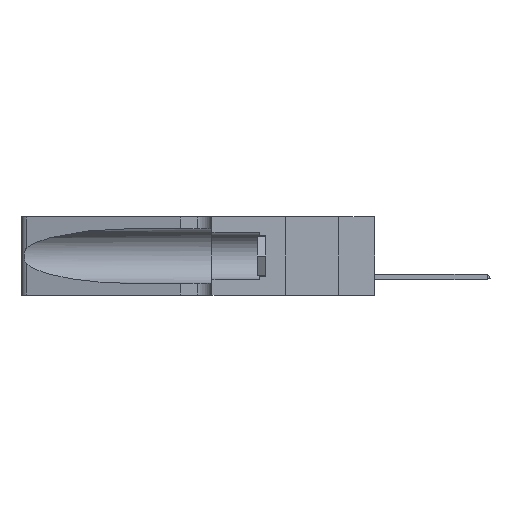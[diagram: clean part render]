
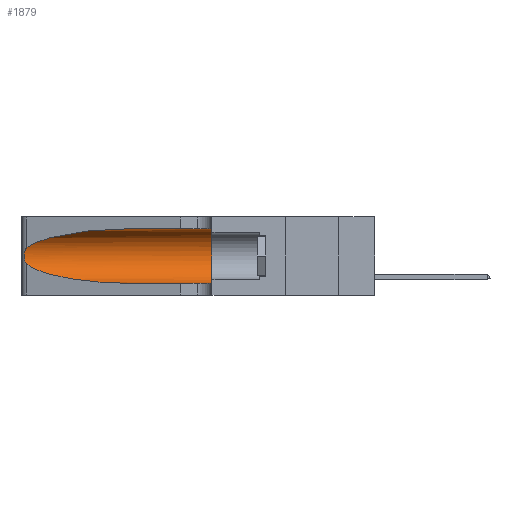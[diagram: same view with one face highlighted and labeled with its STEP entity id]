
A CAD part, left-side view. The second image highlights one B-rep face of the part: STEP entity #1879.
In plain terms, the highlighted cylindrical face has radius 3.308 mm (diameter 6.617 mm), a partial arc.
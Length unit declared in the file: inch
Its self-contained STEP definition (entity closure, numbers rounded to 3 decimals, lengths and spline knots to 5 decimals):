
#87 = ORIENTED_EDGE ( 'NONE', *, *, #16182, .T. ) ;
#844 = CARTESIAN_POINT ( 'NONE',  ( 0.1305, 0.72297, 0.31525 ) ) ;
#902 = CARTESIAN_POINT ( 'NONE',  ( 0.25639, 1.23184, 0.21858 ) ) ;
#1334 = CARTESIAN_POINT ( 'NONE',  ( 0.1305, 0.35, 0.185 ) ) ;
#1475 = CARTESIAN_POINT ( 'NONE',  ( 0.1305, 1.61858, 0.05475 ) ) ;
#1653 = CARTESIAN_POINT ( 'NONE',  ( 0.25487, 1.22718, 0.22369 ) ) ;
#1822 = CARTESIAN_POINT ( 'NONE',  ( 0.1305, 0.35, 0.05475 ) ) ;
#1879 = ADVANCED_FACE ( 'NONE', ( #11630 ), #5560, .F. ) ;
#2768 = CARTESIAN_POINT ( 'NONE',  ( 0.25854, 1.2359, 0.20912 ) ) ;
#2999 = CARTESIAN_POINT ( 'NONE',  ( 0.25487, 1.22718, 0.22369 ) ) ;
#3214 = DIRECTION ( 'NONE',  ( 0., 1., 0. ) ) ;
#3423 = CARTESIAN_POINT ( 'NONE',  ( 0.25555, 1.22993, 0.14849 ) ) ;
#4198 = CARTESIAN_POINT ( 'NONE',  ( 0.25487, 1.22718, 0.14631 ) ) ;
#4410 = DIRECTION ( 'NONE',  ( 0., -1., 0. ) ) ;
#4903 = B_SPLINE_CURVE_WITH_KNOTS ( 'NONE', 3,
 ( #1653, #14313, #902, #13885, #2768, #15764, #6525, #19483, #14277, #20325, #13732, #17566, #3423, #6770 ),
 .UNSPECIFIED., .F., .F.,
 ( 4, 2, 2, 2, 2, 2, 4 ),
 ( 0., 0.00027, 0.00053, 0.00107, 0.0016, 0.00187, 0.00214 ),
 .UNSPECIFIED. ) ;
#5290 = VERTEX_POINT ( 'NONE', #15614 ) ;
#5560 = CYLINDRICAL_SURFACE ( 'NONE', #12633, 0.13025 ) ;
#5692 = AXIS2_PLACEMENT_3D ( 'NONE', #1334, #3214, #14307 ) ;
#5736 = EDGE_CURVE ( 'NONE', #14809, #5290, #17049, .T. ) ;
#5942 = DIRECTION ( 'NONE',  ( 0., 0., -1. ) ) ;
#6525 = CARTESIAN_POINT ( 'NONE',  ( 0.26075, 1.23896, 0.19203 ) ) ;
#6770 = CARTESIAN_POINT ( 'NONE',  ( 0.25487, 1.22718, 0.14631 ) ) ;
#6805 = CARTESIAN_POINT ( 'NONE',  ( 0.1305, 0.72297, 0.31525 ) ) ;
#8408 = ORIENTED_EDGE ( 'NONE', *, *, #16212, .T. ) ;
#8660 = CARTESIAN_POINT ( 'NONE',  ( 0.25487, 1.22718, 0.14631 ) ) ;
#9199 = EDGE_CURVE ( 'NONE', #14809, #20631, #14669, .T. ) ;
#9247 = VECTOR ( 'NONE', #12027, 39.37008 ) ;
#9917 = CARTESIAN_POINT ( 'NONE',  ( 0.1305, 1.61858, 0.31525 ) ) ;
#11327 = VERTEX_POINT ( 'NONE', #1822 ) ;
#11409 = CARTESIAN_POINT ( 'NONE',  ( 0.18966, 0.96281, 0.05475 ) ) ;
#11630 = FACE_OUTER_BOUND ( 'NONE', #22243, .T. ) ;
#11974 = CARTESIAN_POINT ( 'NONE',  ( 0.1305, 0.72297, 0.05475 ) ) ;
#12027 = DIRECTION ( 'NONE',  ( 0., -1., 0. ) ) ;
#12633 = AXIS2_PLACEMENT_3D ( 'NONE', #15256, #13084, #5942 ) ;
#13069 = ORIENTED_EDGE ( 'NONE', *, *, #15015, .F. ) ;
#13084 = DIRECTION ( 'NONE',  ( 0., -1., 0. ) ) ;
#13732 = CARTESIAN_POINT ( 'NONE',  ( 0.25789, 1.23486, 0.15765 ) ) ;
#13885 = CARTESIAN_POINT ( 'NONE',  ( 0.25787, 1.23484, 0.2124 ) ) ;
#14147 = LINE ( 'NONE', #1475, #9247 ) ;
#14175 = CARTESIAN_POINT ( 'NONE',  ( 0.1305, 0.72297, 0.05475 ) ) ;
#14277 = CARTESIAN_POINT ( 'NONE',  ( 0.26017, 1.23833, 0.17102 ) ) ;
#14307 = DIRECTION ( 'NONE',  ( 0., 0., 1. ) ) ;
#14308 = CARTESIAN_POINT ( 'NONE',  ( 0.18966, 0.96281, 0.31525 ) ) ;
#14313 = CARTESIAN_POINT ( 'NONE',  ( 0.25555, 1.22994, 0.2215 ) ) ;
#14383 = CARTESIAN_POINT ( 'NONE',  ( 0.2373, 1.15595, 0.28018 ) ) ;
#14669 =( BOUNDED_CURVE ( )  B_SPLINE_CURVE ( 3, ( #6805, #14308, #14383, #19768 ),
 .UNSPECIFIED., .F., .F. ) 
 B_SPLINE_CURVE_WITH_KNOTS ( ( 4, 4 ),
 ( 1.5708, 2.84003 ),
 .UNSPECIFIED. ) 
 CURVE ( )  GEOMETRIC_REPRESENTATION_ITEM ( )  RATIONAL_B_SPLINE_CURVE ( ( 1., 0.87, 0.87, 1. ) ) 
 REPRESENTATION_ITEM ( '' )  );
#14809 = VERTEX_POINT ( 'NONE', #844 ) ;
#15015 = EDGE_CURVE ( 'NONE', #5290, #11327, #23698, .T. ) ;
#15053 = CARTESIAN_POINT ( 'NONE',  ( 0.2373, 1.15595, 0.08982 ) ) ;
#15256 = CARTESIAN_POINT ( 'NONE',  ( 0.1305, 1.61858, 0.185 ) ) ;
#15432 =( BOUNDED_CURVE ( )  B_SPLINE_CURVE ( 3, ( #8660, #15053, #11409, #11974 ),
 .UNSPECIFIED., .F., .T. ) 
 B_SPLINE_CURVE_WITH_KNOTS ( ( 4, 4 ),
 ( 3.44316, 4.71239 ),
 .UNSPECIFIED. ) 
 CURVE ( )  GEOMETRIC_REPRESENTATION_ITEM ( )  RATIONAL_B_SPLINE_CURVE ( ( 1., 0.87, 0.87, 1. ) ) 
 REPRESENTATION_ITEM ( '' )  );
#15499 = ORIENTED_EDGE ( 'NONE', *, *, #5736, .F. ) ;
#15614 = CARTESIAN_POINT ( 'NONE',  ( 0.1305, 0.35, 0.31525 ) ) ;
#15764 = CARTESIAN_POINT ( 'NONE',  ( 0.26018, 1.23835, 0.19895 ) ) ;
#16177 = EDGE_CURVE ( 'NONE', #20631, #23082, #4903, .T. ) ;
#16182 = EDGE_CURVE ( 'NONE', #17583, #11327, #14147, .T. ) ;
#16212 = EDGE_CURVE ( 'NONE', #23082, #17583, #15432, .T. ) ;
#17049 = LINE ( 'NONE', #9917, #21955 ) ;
#17566 = CARTESIAN_POINT ( 'NONE',  ( 0.25639, 1.23186, 0.15144 ) ) ;
#17583 = VERTEX_POINT ( 'NONE', #14175 ) ;
#18142 = ORIENTED_EDGE ( 'NONE', *, *, #9199, .T. ) ;
#19483 = CARTESIAN_POINT ( 'NONE',  ( 0.26075, 1.23896, 0.178 ) ) ;
#19768 = CARTESIAN_POINT ( 'NONE',  ( 0.25487, 1.22718, 0.22369 ) ) ;
#20325 = CARTESIAN_POINT ( 'NONE',  ( 0.25856, 1.23593, 0.16098 ) ) ;
#20631 = VERTEX_POINT ( 'NONE', #2999 ) ;
#21955 = VECTOR ( 'NONE', #4410, 39.37008 ) ;
#22243 = EDGE_LOOP ( 'NONE', ( #18142, #22377, #8408, #87, #13069, #15499 ) ) ;
#22377 = ORIENTED_EDGE ( 'NONE', *, *, #16177, .T. ) ;
#23082 = VERTEX_POINT ( 'NONE', #4198 ) ;
#23698 = CIRCLE ( 'NONE', #5692, 0.13025 ) ;
